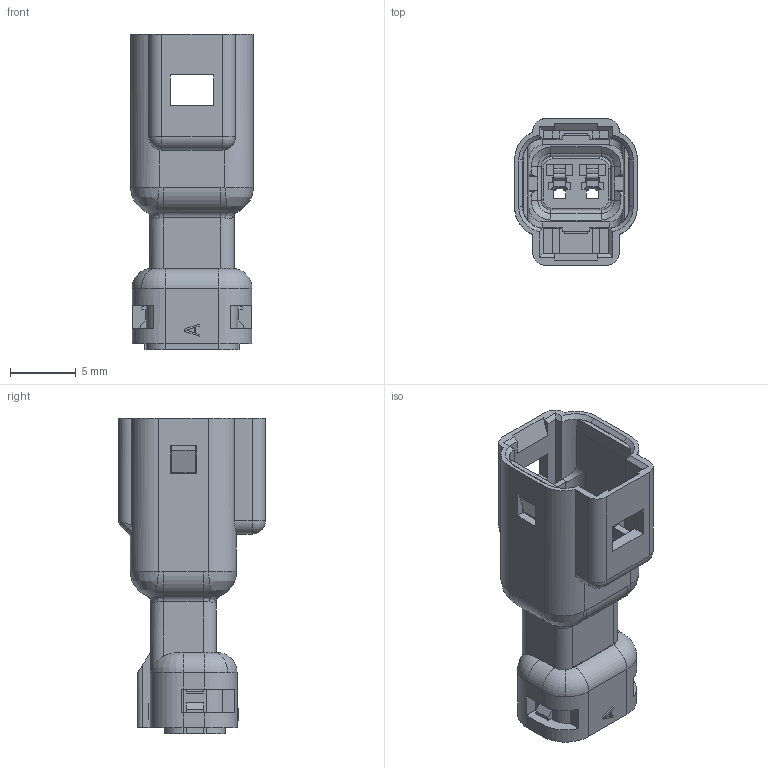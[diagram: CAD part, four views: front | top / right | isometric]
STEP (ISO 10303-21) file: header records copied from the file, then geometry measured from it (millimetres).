
FILE_DESCRIPTION (( 'STEP AP203' ), '1' );
FILE_NAME ('560-002-000-511.STEP', '2020-07-24T15:18:09', ( '' ), ( '' ), 'SwSTEP 2.0', 'SolidWorks 2020', '' );
FILE_SCHEMA (( 'CONFIG_CONTROL_DESIGN' ));
Length unit declared in the file: millimetre
Products named in the file (7): 560-002-000-511; MALE-HOUSING-2POS_ORANGE; INSULATOR-2POS; FACIAL-SEAL-2POS; REAR-GASKET-2POS_ORANGE; INTERNAL-WIRE-SEAL-2POS
Assembly tree (6 placements, depth 3):
  560-002-000-511
    560-002-000-511
      MALE-HOUSING-2POS_ORANGE
      INTERNAL-WIRE-SEAL-2POS
      FACIAL-SEAL-2POS
      INSULATOR-2POS
      REAR-GASKET-2POS_ORANGE
Bounding box: 9.3 x 11.15 x 23.98 mm (x, y, z)
Volume: 900.4 mm3; surface area: 2421 mm2
Topology: 5 solids, 5 shells, 895 faces, 2291 edges, 1410 vertices
Faces by surface type: plane 495, cylinder 209, torus 97, cone 62, bspline 30, sphere 2
Entity records: 29403 total; most frequent: CARTESIAN_POINT 7121, ORIENTED_EDGE 4578, DIRECTION 4432, EDGE_CURVE 2289, LINE 1534, VECTOR 1534, AXIS2_PLACEMENT_3D 1449, VERTEX_POINT 1410
